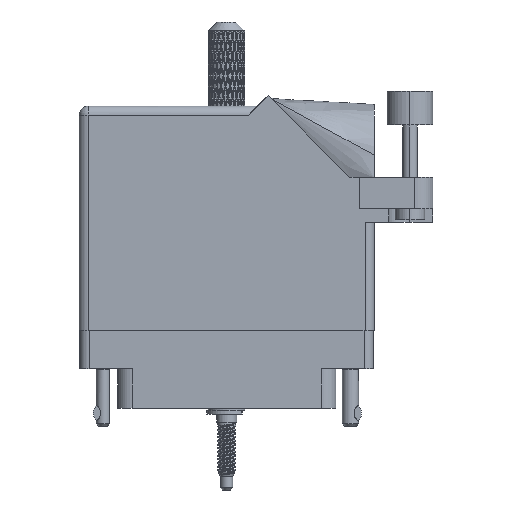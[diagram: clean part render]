
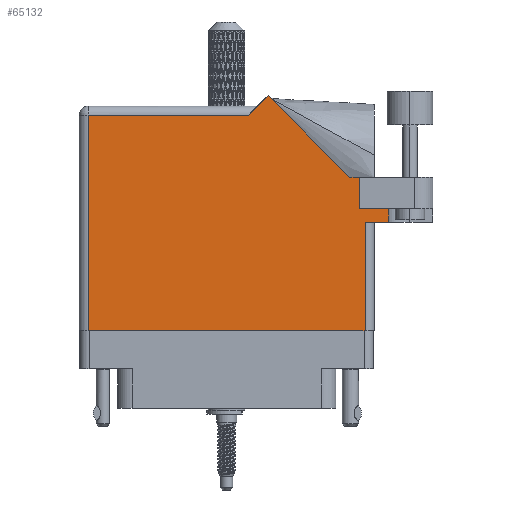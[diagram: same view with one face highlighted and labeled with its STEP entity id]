
A CAD part, front view. The second image highlights one B-rep face of the part: STEP entity #65132.
In plain terms, the highlighted face is planar.
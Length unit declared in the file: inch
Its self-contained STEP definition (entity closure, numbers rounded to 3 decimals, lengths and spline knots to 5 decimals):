
#533 = EDGE_CURVE ( 'NONE', #47159, #5984, #60243, .T. ) ;
#2423 = CARTESIAN_POINT ( 'NONE',  ( 1.91, 0.831, 0. ) ) ;
#4891 = VERTEX_POINT ( 'NONE', #89228 ) ;
#5451 = VECTOR ( 'NONE', #103791, 39.37008 ) ;
#5984 = VERTEX_POINT ( 'NONE', #71989 ) ;
#7012 = PLANE ( 'NONE',  #24333 ) ;
#8753 = LINE ( 'NONE', #76359, #59329 ) ;
#10890 = CARTESIAN_POINT ( 'NONE',  ( 1.91, 0.831, 0. ) ) ;
#11225 = VERTEX_POINT ( 'NONE', #78624 ) ;
#15370 = VERTEX_POINT ( 'NONE', #45743 ) ;
#18341 = LINE ( 'NONE', #2423, #66298 ) ;
#18555 = LINE ( 'NONE', #24692, #66518 ) ;
#18701 = CARTESIAN_POINT ( 'NONE',  ( 1.84442, 1.044, 0. ) ) ;
#19793 = DIRECTION ( 'NONE',  ( 0., 1., 0. ) ) ;
#20485 = ORIENTED_EDGE ( 'NONE', *, *, #93396, .T. ) ;
#20602 = LINE ( 'NONE', #18701, #61914 ) ;
#22542 = EDGE_CURVE ( 'NONE', #35081, #35366, #26005, .T. ) ;
#22849 = ORIENTED_EDGE ( 'NONE', *, *, #90849, .T. ) ;
#23138 = CARTESIAN_POINT ( 'NONE',  ( 2.1115, 1.16177, 0. ) ) ;
#24333 = AXIS2_PLACEMENT_3D ( 'NONE', #75107, #66890, #24470 ) ;
#24470 = DIRECTION ( 'NONE',  ( -1., 0., 0. ) ) ;
#24692 = CARTESIAN_POINT ( 'NONE',  ( 1.948, 0.737, 0. ) ) ;
#26005 = LINE ( 'NONE', #79867, #45971 ) ;
#27704 = DIRECTION ( 'NONE',  ( 1., 0., 0. ) ) ;
#28164 = EDGE_LOOP ( 'NONE', ( #65809, #22849, #93508, #28497, #84727, #94981, #20485, #60841, #46036, #82710, #90732 ) ) ;
#28497 = ORIENTED_EDGE ( 'NONE', *, *, #85829, .F. ) ;
#31022 = VECTOR ( 'NONE', #19793, 39.37008 ) ;
#35081 = VERTEX_POINT ( 'NONE', #61561 ) ;
#35366 = VERTEX_POINT ( 'NONE', #110009 ) ;
#35434 = EDGE_CURVE ( 'NONE', #45951, #4891, #8753, .T. ) ;
#40292 = EDGE_CURVE ( 'NONE', #72881, #67542, #108034, .T. ) ;
#41067 = CARTESIAN_POINT ( 'NONE',  ( 2.1115, 0.737, 0. ) ) ;
#44640 = VECTOR ( 'NONE', #101186, 39.37008 ) ;
#44962 = CARTESIAN_POINT ( 'NONE',  ( 0.062, 0., 0. ) ) ;
#45317 = DIRECTION ( 'NONE',  ( 0., -1., 0. ) ) ;
#45743 = CARTESIAN_POINT ( 'NONE',  ( 2.1115, 0.831, 0. ) ) ;
#45951 = VERTEX_POINT ( 'NONE', #91027 ) ;
#45971 = VECTOR ( 'NONE', #105283, 39.37008 ) ;
#46036 = ORIENTED_EDGE ( 'NONE', *, *, #106746, .T. ) ;
#47159 = VERTEX_POINT ( 'NONE', #51911 ) ;
#48027 = DIRECTION ( 'NONE',  ( -0.707, -0.707, 0. ) ) ;
#48291 = EDGE_CURVE ( 'NONE', #11225, #64473, #20602, .T. ) ;
#50903 = LINE ( 'NONE', #23138, #102859 ) ;
#51165 = VECTOR ( 'NONE', #48027, 39.37008 ) ;
#51911 = CARTESIAN_POINT ( 'NONE',  ( 1.91, 0.831, 0. ) ) ;
#58099 = DIRECTION ( 'NONE',  ( 0., -1., 0. ) ) ;
#59329 = VECTOR ( 'NONE', #68172, 39.37008 ) ;
#60243 = LINE ( 'NONE', #10890, #31022 ) ;
#60841 = ORIENTED_EDGE ( 'NONE', *, *, #48291, .T. ) ;
#61561 = CARTESIAN_POINT ( 'NONE',  ( 1.155, 1.468, 0. ) ) ;
#61830 = FACE_OUTER_BOUND ( 'NONE', #28164, .T. ) ;
#61914 = VECTOR ( 'NONE', #86861, 39.37008 ) ;
#64473 = VERTEX_POINT ( 'NONE', #101963 ) ;
#65132 = ADVANCED_FACE ( 'NONE', ( #61830 ), #7012, .F. ) ;
#65809 = ORIENTED_EDGE ( 'NONE', *, *, #35434, .T. ) ;
#66029 = DIRECTION ( 'NONE',  ( 0., 1., 0. ) ) ;
#66298 = VECTOR ( 'NONE', #27704, 39.37008 ) ;
#66518 = VECTOR ( 'NONE', #66029, 39.37008 ) ;
#66890 = DIRECTION ( 'NONE',  ( 0., 0., -1. ) ) ;
#67542 = VERTEX_POINT ( 'NONE', #41067 ) ;
#67979 = EDGE_CURVE ( 'NONE', #35366, #45951, #86878, .T. ) ;
#68172 = DIRECTION ( 'NONE',  ( 1., 0., 0. ) ) ;
#71989 = CARTESIAN_POINT ( 'NONE',  ( 1.91, 1.044, 0. ) ) ;
#72881 = VERTEX_POINT ( 'NONE', #84564 ) ;
#75107 = CARTESIAN_POINT ( 'NONE',  ( 0., 1.53, 0. ) ) ;
#76359 = CARTESIAN_POINT ( 'NONE',  ( 0., 0., 0. ) ) ;
#78624 = CARTESIAN_POINT ( 'NONE',  ( 1.84442, 1.044, 0. ) ) ;
#79867 = CARTESIAN_POINT ( 'NONE',  ( 0., 1.468, 0. ) ) ;
#82710 = ORIENTED_EDGE ( 'NONE', *, *, #22542, .T. ) ;
#84564 = CARTESIAN_POINT ( 'NONE',  ( 1.948, 0.737, 0. ) ) ;
#84727 = ORIENTED_EDGE ( 'NONE', *, *, #108986, .F. ) ;
#85829 = EDGE_CURVE ( 'NONE', #15370, #67542, #50903, .T. ) ;
#86861 = DIRECTION ( 'NONE',  ( -0.707, 0.707, 0. ) ) ;
#86878 = LINE ( 'NONE', #44962, #102944 ) ;
#89228 = CARTESIAN_POINT ( 'NONE',  ( 1.948, 0., 0. ) ) ;
#90732 = ORIENTED_EDGE ( 'NONE', *, *, #67979, .T. ) ;
#90849 = EDGE_CURVE ( 'NONE', #4891, #72881, #18555, .T. ) ;
#91027 = CARTESIAN_POINT ( 'NONE',  ( 0.062, 0., 0. ) ) ;
#91305 = LINE ( 'NONE', #93288, #44640 ) ;
#92480 = LINE ( 'NONE', #97955, #51165 ) ;
#93288 = CARTESIAN_POINT ( 'NONE',  ( 2.41, 1.044, 0. ) ) ;
#93396 = EDGE_CURVE ( 'NONE', #5984, #11225, #91305, .T. ) ;
#93508 = ORIENTED_EDGE ( 'NONE', *, *, #40292, .T. ) ;
#94981 = ORIENTED_EDGE ( 'NONE', *, *, #533, .T. ) ;
#97955 = CARTESIAN_POINT ( 'NONE',  ( 1.217, 1.53, 0. ) ) ;
#101186 = DIRECTION ( 'NONE',  ( -1., 0., 0. ) ) ;
#101963 = CARTESIAN_POINT ( 'NONE',  ( 1.28771, 1.60071, 0. ) ) ;
#102859 = VECTOR ( 'NONE', #58099, 39.37008 ) ;
#102944 = VECTOR ( 'NONE', #45317, 39.37008 ) ;
#103073 = CARTESIAN_POINT ( 'NONE',  ( 2.01, 0.737, 0. ) ) ;
#103791 = DIRECTION ( 'NONE',  ( 1., 0., 0. ) ) ;
#105283 = DIRECTION ( 'NONE',  ( -1., 0., 0. ) ) ;
#106746 = EDGE_CURVE ( 'NONE', #64473, #35081, #92480, .T. ) ;
#108034 = LINE ( 'NONE', #103073, #5451 ) ;
#108986 = EDGE_CURVE ( 'NONE', #47159, #15370, #18341, .T. ) ;
#110009 = CARTESIAN_POINT ( 'NONE',  ( 0.062, 1.468, 0. ) ) ;
